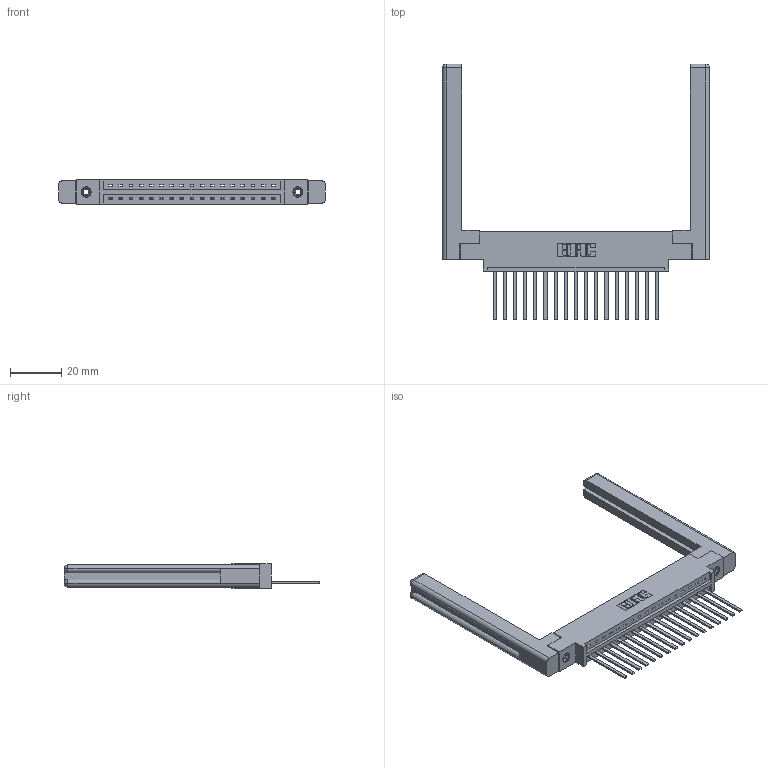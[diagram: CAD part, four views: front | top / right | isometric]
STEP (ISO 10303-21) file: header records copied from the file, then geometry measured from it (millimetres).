
FILE_DESCRIPTION (( 'STEP AP203' ), '1' );
FILE_NAME ('387-017-544-658.STEP', '2019-10-02T19:38:34', ( '' ), ( '' ), 'SwSTEP 2.0', 'SolidWorks 2016', '' );
FILE_SCHEMA (( 'CONFIG_CONTROL_DESIGN' ));
Length unit declared in the file: inch
Products named in the file (5): 337 Part_0.170 Offset - 0.156 Dia-TI; 307-220-058; 345-250-001_345-250-001-102; 345-292-001_345-293-144; 387-017-544-658
Assembly tree (22 placements, depth 2):
  387-017-544-658
    337 Part_0.170 Offset - 0.156 Dia-TI
    345-292-001_345-293-144  x17
    345-250-001_345-250-001-102  x2
    307-220-058  x2
Bounding box: 103.99 x 99.7 x 9.4 mm (x, y, z)
Volume: 17736.4 mm3; surface area: 16745.3 mm2
Topology: 22 solids, 22 shells, 1212 faces, 3567 edges, 2342 vertices
Faces by surface type: plane 872, cylinder 316, cone 12, torus 12
Entity records: 18452 total; most frequent: CARTESIAN_POINT 3212, ORIENTED_EDGE 3104, DIRECTION 2770, EDGE_CURVE 1552, VECTOR 1380, LINE 1380, VERTEX_POINT 1026, AXIS2_PLACEMENT_3D 695
